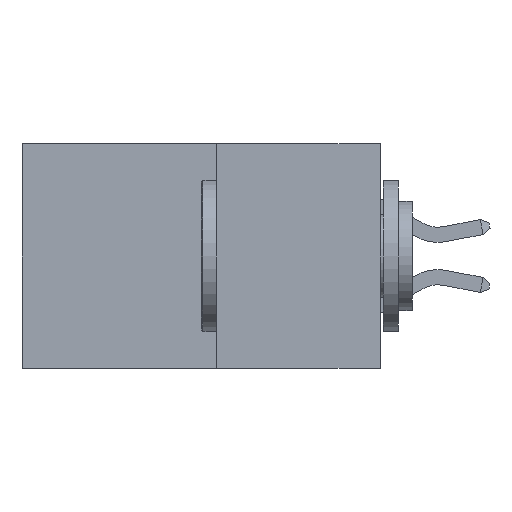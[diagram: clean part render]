
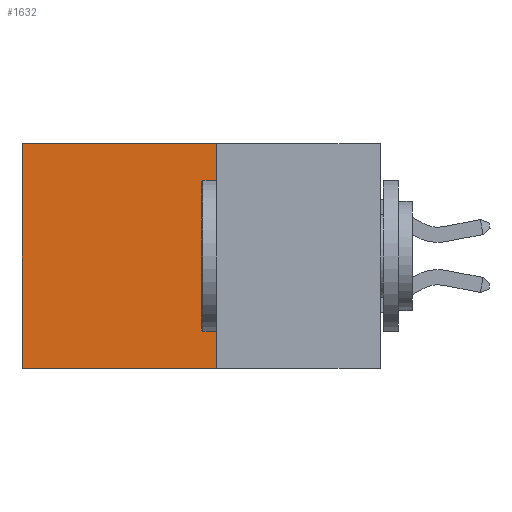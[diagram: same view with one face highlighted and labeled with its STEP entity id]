
A CAD part, left-side view. The second image highlights one B-rep face of the part: STEP entity #1632.
In plain terms, the highlighted planar face has unit normal (-1, 0, 0).
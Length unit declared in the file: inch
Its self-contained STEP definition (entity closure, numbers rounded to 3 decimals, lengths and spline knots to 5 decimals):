
#265 = EDGE_CURVE ( 'NONE', #298, #20535, #21127, .T. ) ;
#289 = CARTESIAN_POINT ( 'NONE',  ( 0.277, 0.59, -0.37 ) ) ;
#298 = VERTEX_POINT ( 'NONE', #33280 ) ;
#341 = LINE ( 'NONE', #27920, #13149 ) ;
#1600 = ORIENTED_EDGE ( 'NONE', *, *, #265, .F. ) ;
#1632 = ADVANCED_FACE ( 'NONE', ( #29047 ), #32442, .F. ) ;
#3734 = LINE ( 'NONE', #23497, #32493 ) ;
#4457 = CARTESIAN_POINT ( 'NONE',  ( 0.277, 0.59, 0. ) ) ;
#5522 = EDGE_CURVE ( 'NONE', #32083, #29167, #15409, .T. ) ;
#6630 = VECTOR ( 'NONE', #29467, 39.37008 ) ;
#9320 = CARTESIAN_POINT ( 'NONE',  ( 0.277, 0.27, -0.37 ) ) ;
#10163 = CARTESIAN_POINT ( 'NONE',  ( 0.277, 0.59, -0.37 ) ) ;
#10589 = DIRECTION ( 'NONE',  ( 0., 0., -1. ) ) ;
#12569 = DIRECTION ( 'NONE',  ( 0., 1., 0. ) ) ;
#13149 = VECTOR ( 'NONE', #14414, 39.37008 ) ;
#14414 = DIRECTION ( 'NONE',  ( 0., 1., 0. ) ) ;
#14602 = ORIENTED_EDGE ( 'NONE', *, *, #5522, .T. ) ;
#15409 = LINE ( 'NONE', #10163, #28962 ) ;
#19723 = EDGE_LOOP ( 'NONE', ( #14602, #29779, #1600, #26341 ) ) ;
#19906 = EDGE_CURVE ( 'NONE', #298, #32083, #3734, .T. ) ;
#20535 = VERTEX_POINT ( 'NONE', #23228 ) ;
#21127 = LINE ( 'NONE', #9320, #6630 ) ;
#23228 = CARTESIAN_POINT ( 'NONE',  ( 0.277, 0.27, -0.37 ) ) ;
#23497 = CARTESIAN_POINT ( 'NONE',  ( 0.277, 0.27, 0. ) ) ;
#26341 = ORIENTED_EDGE ( 'NONE', *, *, #19906, .T. ) ;
#27085 = EDGE_CURVE ( 'NONE', #20535, #29167, #341, .T. ) ;
#27920 = CARTESIAN_POINT ( 'NONE',  ( 0.277, 0.27, -0.37 ) ) ;
#28962 = VECTOR ( 'NONE', #10589, 39.37008 ) ;
#29047 = FACE_OUTER_BOUND ( 'NONE', #19723, .T. ) ;
#29167 = VERTEX_POINT ( 'NONE', #289 ) ;
#29467 = DIRECTION ( 'NONE',  ( 0., 0., -1. ) ) ;
#29779 = ORIENTED_EDGE ( 'NONE', *, *, #27085, .F. ) ;
#32083 = VERTEX_POINT ( 'NONE', #4457 ) ;
#32291 = CARTESIAN_POINT ( 'NONE',  ( 0.277, 0.27, -0.37 ) ) ;
#32372 = DIRECTION ( 'NONE',  ( 1., 0., 0. ) ) ;
#32442 = PLANE ( 'NONE',  #32914 ) ;
#32493 = VECTOR ( 'NONE', #12569, 39.37008 ) ;
#32914 = AXIS2_PLACEMENT_3D ( 'NONE', #32291, #32372, #33849 ) ;
#33280 = CARTESIAN_POINT ( 'NONE',  ( 0.277, 0.27, 0. ) ) ;
#33849 = DIRECTION ( 'NONE',  ( 0., 0., -1. ) ) ;
